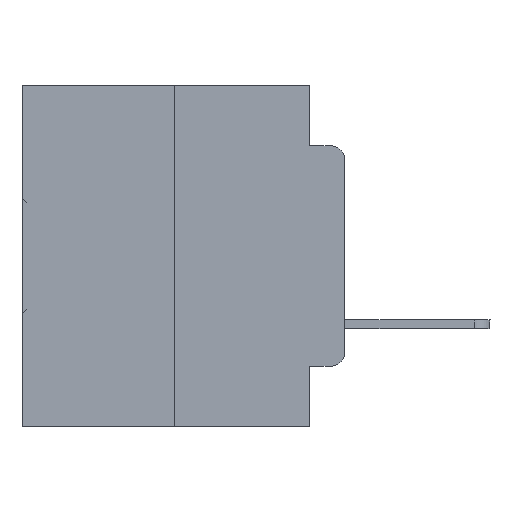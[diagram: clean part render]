
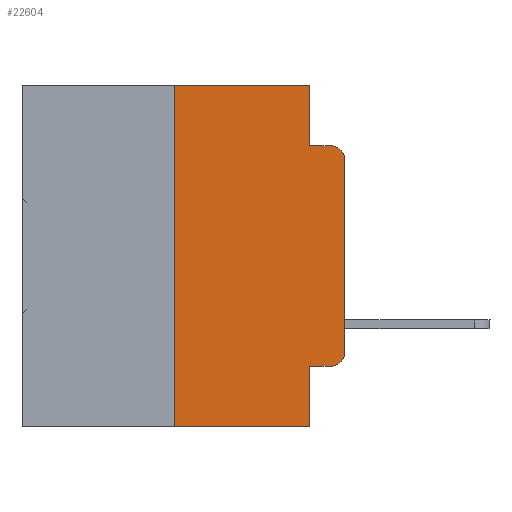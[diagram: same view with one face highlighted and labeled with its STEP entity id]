
A CAD part, left-side view. The second image highlights one B-rep face of the part: STEP entity #22604.
In plain terms, the highlighted planar face has unit normal (-1, 0, 0).
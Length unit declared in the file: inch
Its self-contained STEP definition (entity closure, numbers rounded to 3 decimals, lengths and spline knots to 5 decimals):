
#1304 = ORIENTED_EDGE ( 'NONE', *, *, #4444, .F. ) ;
#1401 = VERTEX_POINT ( 'NONE', #21689 ) ;
#1880 = VECTOR ( 'NONE', #31049, 39.37008 ) ;
#1959 = CARTESIAN_POINT ( 'NONE',  ( 0., 0., 0. ) ) ;
#1980 = EDGE_LOOP ( 'NONE', ( #16886, #4980, #1304, #13332, #25015, #3830, #11841, #18938, #27416, #30012 ) ) ;
#2044 = CARTESIAN_POINT ( 'NONE',  ( 0., 0.02, -0.0885 ) ) ;
#2601 = DIRECTION ( 'NONE',  ( 0., 0., -1. ) ) ;
#2777 = CARTESIAN_POINT ( 'NONE',  ( 0., 0.051, -0.4115 ) ) ;
#3070 = VERTEX_POINT ( 'NONE', #13471 ) ;
#3830 = ORIENTED_EDGE ( 'NONE', *, *, #11144, .F. ) ;
#4081 = AXIS2_PLACEMENT_3D ( 'NONE', #17616, #19958, #2601 ) ;
#4444 = EDGE_CURVE ( 'NONE', #20656, #6578, #15852, .T. ) ;
#4750 = CARTESIAN_POINT ( 'NONE',  ( 0., 0.25, 0. ) ) ;
#4980 = ORIENTED_EDGE ( 'NONE', *, *, #19104, .T. ) ;
#5516 = CARTESIAN_POINT ( 'NONE',  ( 0., 0.051, -0.0885 ) ) ;
#5665 = EDGE_CURVE ( 'NONE', #17705, #1401, #32822, .T. ) ;
#6578 = VERTEX_POINT ( 'NONE', #2044 ) ;
#6865 = DIRECTION ( 'NONE',  ( 0., -1., 0. ) ) ;
#7112 = CARTESIAN_POINT ( 'NONE',  ( 0., 0.051, 0. ) ) ;
#7269 = VERTEX_POINT ( 'NONE', #27335 ) ;
#7786 = EDGE_CURVE ( 'NONE', #16141, #23673, #13119, .T. ) ;
#8150 = LINE ( 'NONE', #20845, #1880 ) ;
#8479 = DIRECTION ( 'NONE',  ( 0., 0., -1. ) ) ;
#8564 = CARTESIAN_POINT ( 'NONE',  ( 0., 0., -0.3915 ) ) ;
#9271 = AXIS2_PLACEMENT_3D ( 'NONE', #11898, #19558, #29768 ) ;
#10614 = VECTOR ( 'NONE', #6865, 39.37008 ) ;
#10954 = DIRECTION ( 'NONE',  ( 0., -1., 0. ) ) ;
#11144 = EDGE_CURVE ( 'NONE', #32524, #16345, #17428, .T. ) ;
#11294 = VECTOR ( 'NONE', #29840, 39.37008 ) ;
#11841 = ORIENTED_EDGE ( 'NONE', *, *, #22392, .T. ) ;
#11898 = CARTESIAN_POINT ( 'NONE',  ( 0., 0.02, -0.1085 ) ) ;
#12005 = VECTOR ( 'NONE', #18528, 39.37008 ) ;
#12080 = CARTESIAN_POINT ( 'NONE',  ( 0., 0.051, -0.4115 ) ) ;
#12780 = CARTESIAN_POINT ( 'NONE',  ( 0., 0.25, -0.5 ) ) ;
#13119 = LINE ( 'NONE', #2777, #32419 ) ;
#13169 = CIRCLE ( 'NONE', #4081, 0.02 ) ;
#13332 = ORIENTED_EDGE ( 'NONE', *, *, #16906, .F. ) ;
#13471 = CARTESIAN_POINT ( 'NONE',  ( 0., 0.051, -0.5 ) ) ;
#13977 = FACE_OUTER_BOUND ( 'NONE', #1980, .T. ) ;
#14545 = CARTESIAN_POINT ( 'NONE',  ( 0., 0.473, 0. ) ) ;
#14922 = DIRECTION ( 'NONE',  ( 0., 0., 1. ) ) ;
#15072 = CARTESIAN_POINT ( 'NONE',  ( 0., 0.25, 0. ) ) ;
#15852 = LINE ( 'NONE', #5516, #12005 ) ;
#16061 = EDGE_CURVE ( 'NONE', #16141, #3070, #16915, .T. ) ;
#16141 = VERTEX_POINT ( 'NONE', #12080 ) ;
#16345 = VERTEX_POINT ( 'NONE', #15072 ) ;
#16470 = CARTESIAN_POINT ( 'NONE',  ( 0., 0.473, 0. ) ) ;
#16886 = ORIENTED_EDGE ( 'NONE', *, *, #5665, .T. ) ;
#16906 = EDGE_CURVE ( 'NONE', #7269, #20656, #19962, .T. ) ;
#16915 = LINE ( 'NONE', #22091, #31526 ) ;
#17428 = LINE ( 'NONE', #4750, #30378 ) ;
#17616 = CARTESIAN_POINT ( 'NONE',  ( 0., 0.02, -0.3915 ) ) ;
#17705 = VERTEX_POINT ( 'NONE', #8564 ) ;
#18528 = DIRECTION ( 'NONE',  ( 0., -1., 0. ) ) ;
#18856 = CIRCLE ( 'NONE', #9271, 0.02 ) ;
#18938 = ORIENTED_EDGE ( 'NONE', *, *, #16061, .F. ) ;
#19104 = EDGE_CURVE ( 'NONE', #1401, #6578, #18856, .T. ) ;
#19558 = DIRECTION ( 'NONE',  ( -1., 0., 0. ) ) ;
#19958 = DIRECTION ( 'NONE',  ( -1., 0., 0. ) ) ;
#19962 = LINE ( 'NONE', #7112, #11294 ) ;
#20656 = VERTEX_POINT ( 'NONE', #30244 ) ;
#20845 = CARTESIAN_POINT ( 'NONE',  ( 0., 0.473, -0.5 ) ) ;
#21175 = DIRECTION ( 'NONE',  ( 1., 0., 0. ) ) ;
#21689 = CARTESIAN_POINT ( 'NONE',  ( 0., 0., -0.1085 ) ) ;
#22091 = CARTESIAN_POINT ( 'NONE',  ( 0., 0.051, 0. ) ) ;
#22392 = EDGE_CURVE ( 'NONE', #32524, #3070, #8150, .T. ) ;
#22604 = ADVANCED_FACE ( 'NONE', ( #13977 ), #31546, .F. ) ;
#23673 = VERTEX_POINT ( 'NONE', #24918 ) ;
#24695 = DIRECTION ( 'NONE',  ( 0., 0., 1. ) ) ;
#24918 = CARTESIAN_POINT ( 'NONE',  ( 0., 0.02, -0.4115 ) ) ;
#25015 = ORIENTED_EDGE ( 'NONE', *, *, #27987, .F. ) ;
#25803 = VECTOR ( 'NONE', #24695, 39.37008 ) ;
#25810 = EDGE_CURVE ( 'NONE', #23673, #17705, #13169, .T. ) ;
#27260 = LINE ( 'NONE', #14545, #10614 ) ;
#27335 = CARTESIAN_POINT ( 'NONE',  ( 0., 0.051, 0. ) ) ;
#27416 = ORIENTED_EDGE ( 'NONE', *, *, #7786, .T. ) ;
#27526 = AXIS2_PLACEMENT_3D ( 'NONE', #16470, #21175, #8479 ) ;
#27987 = EDGE_CURVE ( 'NONE', #16345, #7269, #27260, .T. ) ;
#29298 = DIRECTION ( 'NONE',  ( 0., 0., -1. ) ) ;
#29768 = DIRECTION ( 'NONE',  ( 0., 0., -1. ) ) ;
#29840 = DIRECTION ( 'NONE',  ( 0., 0., -1. ) ) ;
#30012 = ORIENTED_EDGE ( 'NONE', *, *, #25810, .T. ) ;
#30244 = CARTESIAN_POINT ( 'NONE',  ( 0., 0.051, -0.0885 ) ) ;
#30378 = VECTOR ( 'NONE', #14922, 39.37008 ) ;
#31049 = DIRECTION ( 'NONE',  ( 0., -1., 0. ) ) ;
#31526 = VECTOR ( 'NONE', #29298, 39.37008 ) ;
#31546 = PLANE ( 'NONE',  #27526 ) ;
#32419 = VECTOR ( 'NONE', #10954, 39.37008 ) ;
#32524 = VERTEX_POINT ( 'NONE', #12780 ) ;
#32822 = LINE ( 'NONE', #1959, #25803 ) ;
